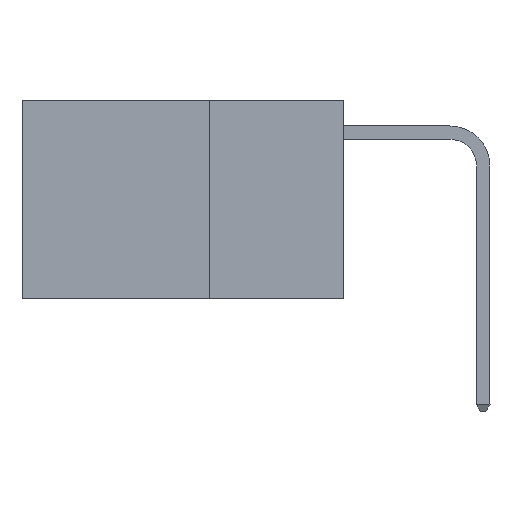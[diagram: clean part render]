
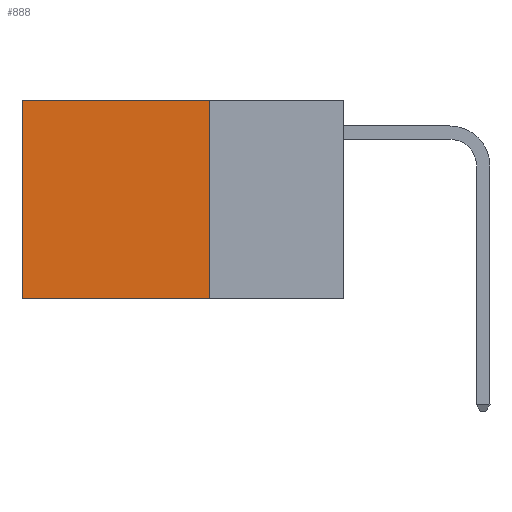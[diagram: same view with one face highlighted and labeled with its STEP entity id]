
A CAD part, left-side view. The second image highlights one B-rep face of the part: STEP entity #888.
In plain terms, the highlighted planar face has unit normal (-1, 0, 0).
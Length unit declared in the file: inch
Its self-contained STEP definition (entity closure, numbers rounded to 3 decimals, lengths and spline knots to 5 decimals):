
#888 = ADVANCED_FACE ( 'NONE', ( #7258 ), #15087, .F. ) ;
#1239 = CARTESIAN_POINT ( 'NONE',  ( 0.2625, 0.25, -0.37 ) ) ;
#1649 = CARTESIAN_POINT ( 'NONE',  ( 0.2625, 0.25, -0.37 ) ) ;
#1810 = VECTOR ( 'NONE', #6726, 39.37008 ) ;
#3165 = ORIENTED_EDGE ( 'NONE', *, *, #9805, .F. ) ;
#3253 = DIRECTION ( 'NONE',  ( 0., 1., 0. ) ) ;
#3265 = EDGE_CURVE ( 'NONE', #4248, #12275, #8782, .T. ) ;
#4248 = VERTEX_POINT ( 'NONE', #12091 ) ;
#5449 = VECTOR ( 'NONE', #8582, 39.37008 ) ;
#6726 = DIRECTION ( 'NONE',  ( 0., 0., -1. ) ) ;
#6978 = CARTESIAN_POINT ( 'NONE',  ( 0.2625, 0.25, 0. ) ) ;
#7258 = FACE_OUTER_BOUND ( 'NONE', #14664, .T. ) ;
#7468 = VERTEX_POINT ( 'NONE', #1239 ) ;
#7764 = ORIENTED_EDGE ( 'NONE', *, *, #3265, .T. ) ;
#8582 = DIRECTION ( 'NONE',  ( 0., 0., -1. ) ) ;
#8782 = LINE ( 'NONE', #19140, #1810 ) ;
#8786 = ORIENTED_EDGE ( 'NONE', *, *, #10844, .T. ) ;
#9805 = EDGE_CURVE ( 'NONE', #7468, #12275, #18642, .T. ) ;
#10844 = EDGE_CURVE ( 'NONE', #12748, #4248, #11040, .T. ) ;
#11040 = LINE ( 'NONE', #11976, #19328 ) ;
#11589 = CARTESIAN_POINT ( 'NONE',  ( 0.2625, 0.25, 0. ) ) ;
#11669 = CARTESIAN_POINT ( 'NONE',  ( 0.2625, 0.6, -0.37 ) ) ;
#11976 = CARTESIAN_POINT ( 'NONE',  ( 0.2625, 0.25, 0. ) ) ;
#12091 = CARTESIAN_POINT ( 'NONE',  ( 0.2625, 0.6, 0. ) ) ;
#12275 = VERTEX_POINT ( 'NONE', #11669 ) ;
#12748 = VERTEX_POINT ( 'NONE', #14363 ) ;
#13785 = LINE ( 'NONE', #6978, #5449 ) ;
#14363 = CARTESIAN_POINT ( 'NONE',  ( 0.2625, 0.25, 0. ) ) ;
#14664 = EDGE_LOOP ( 'NONE', ( #7764, #3165, #15174, #8786 ) ) ;
#15087 = PLANE ( 'NONE',  #16689 ) ;
#15174 = ORIENTED_EDGE ( 'NONE', *, *, #16501, .F. ) ;
#15974 = DIRECTION ( 'NONE',  ( 0., 0., -1. ) ) ;
#16106 = DIRECTION ( 'NONE',  ( 1., 0., 0. ) ) ;
#16501 = EDGE_CURVE ( 'NONE', #12748, #7468, #13785, .T. ) ;
#16651 = DIRECTION ( 'NONE',  ( 0., 1., 0. ) ) ;
#16689 = AXIS2_PLACEMENT_3D ( 'NONE', #11589, #16106, #15974 ) ;
#18164 = VECTOR ( 'NONE', #3253, 39.37008 ) ;
#18642 = LINE ( 'NONE', #1649, #18164 ) ;
#19140 = CARTESIAN_POINT ( 'NONE',  ( 0.2625, 0.6, 0. ) ) ;
#19328 = VECTOR ( 'NONE', #16651, 39.37008 ) ;
